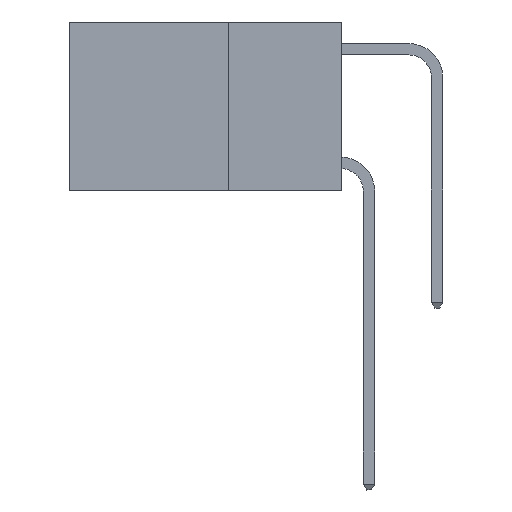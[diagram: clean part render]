
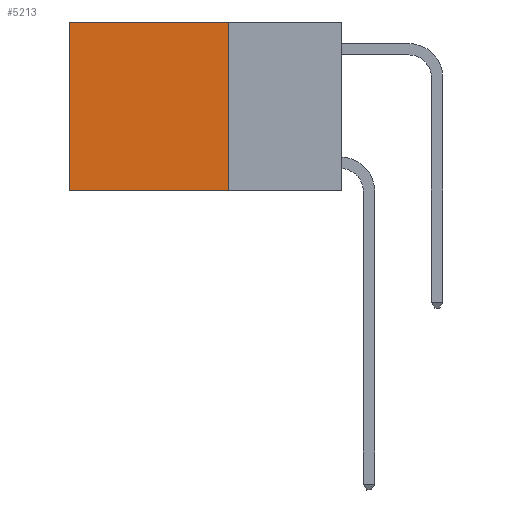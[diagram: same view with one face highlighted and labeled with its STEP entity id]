
A CAD part, left-side view. The second image highlights one B-rep face of the part: STEP entity #5213.
In plain terms, the highlighted planar face has unit normal (-1, 0, 0).
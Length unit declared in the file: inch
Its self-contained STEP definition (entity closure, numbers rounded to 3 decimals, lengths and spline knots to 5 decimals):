
#173 = LINE ( 'NONE', #13111, #7794 ) ;
#300 = DIRECTION ( 'NONE',  ( 0., 1., 0. ) ) ;
#838 = CARTESIAN_POINT ( 'NONE',  ( 0.2625, 0.6, 0. ) ) ;
#1224 = ORIENTED_EDGE ( 'NONE', *, *, #20967, .F. ) ;
#1830 = EDGE_CURVE ( 'NONE', #6200, #15635, #21395, .T. ) ;
#1881 = PLANE ( 'NONE',  #14796 ) ;
#4952 = VECTOR ( 'NONE', #12878, 39.37008 ) ;
#5213 = ADVANCED_FACE ( 'NONE', ( #14581 ), #1881, .F. ) ;
#5404 = VERTEX_POINT ( 'NONE', #5663 ) ;
#5437 = CARTESIAN_POINT ( 'NONE',  ( 0.2625, 0.25, 0. ) ) ;
#5440 = EDGE_LOOP ( 'NONE', ( #6909, #10645, #1224, #8777 ) ) ;
#5548 = DIRECTION ( 'NONE',  ( 1., 0., 0. ) ) ;
#5663 = CARTESIAN_POINT ( 'NONE',  ( 0.2625, 0.25, 0. ) ) ;
#6200 = VERTEX_POINT ( 'NONE', #838 ) ;
#6481 = DIRECTION ( 'NONE',  ( 0., 0., -1. ) ) ;
#6909 = ORIENTED_EDGE ( 'NONE', *, *, #1830, .T. ) ;
#7202 = VECTOR ( 'NONE', #16108, 39.37008 ) ;
#7404 = VERTEX_POINT ( 'NONE', #19516 ) ;
#7794 = VECTOR ( 'NONE', #300, 39.37008 ) ;
#8777 = ORIENTED_EDGE ( 'NONE', *, *, #14043, .T. ) ;
#10645 = ORIENTED_EDGE ( 'NONE', *, *, #22041, .F. ) ;
#10894 = LINE ( 'NONE', #20235, #7202 ) ;
#12878 = DIRECTION ( 'NONE',  ( 0., 1., 0. ) ) ;
#13111 = CARTESIAN_POINT ( 'NONE',  ( 0.2625, 0.25, 0. ) ) ;
#14043 = EDGE_CURVE ( 'NONE', #5404, #6200, #173, .T. ) ;
#14581 = FACE_OUTER_BOUND ( 'NONE', #5440, .T. ) ;
#14663 = VECTOR ( 'NONE', #6481, 39.37008 ) ;
#14796 = AXIS2_PLACEMENT_3D ( 'NONE', #5437, #5548, #21799 ) ;
#15635 = VERTEX_POINT ( 'NONE', #19286 ) ;
#16108 = DIRECTION ( 'NONE',  ( 0., 0., -1. ) ) ;
#16687 = CARTESIAN_POINT ( 'NONE',  ( 0.2625, 0.25, -0.37 ) ) ;
#17278 = CARTESIAN_POINT ( 'NONE',  ( 0.2625, 0.6, 0. ) ) ;
#19286 = CARTESIAN_POINT ( 'NONE',  ( 0.2625, 0.6, -0.37 ) ) ;
#19516 = CARTESIAN_POINT ( 'NONE',  ( 0.2625, 0.25, -0.37 ) ) ;
#20235 = CARTESIAN_POINT ( 'NONE',  ( 0.2625, 0.25, 0. ) ) ;
#20967 = EDGE_CURVE ( 'NONE', #5404, #7404, #10894, .T. ) ;
#21395 = LINE ( 'NONE', #17278, #14663 ) ;
#21799 = DIRECTION ( 'NONE',  ( 0., 0., -1. ) ) ;
#22041 = EDGE_CURVE ( 'NONE', #7404, #15635, #22121, .T. ) ;
#22121 = LINE ( 'NONE', #16687, #4952 ) ;
